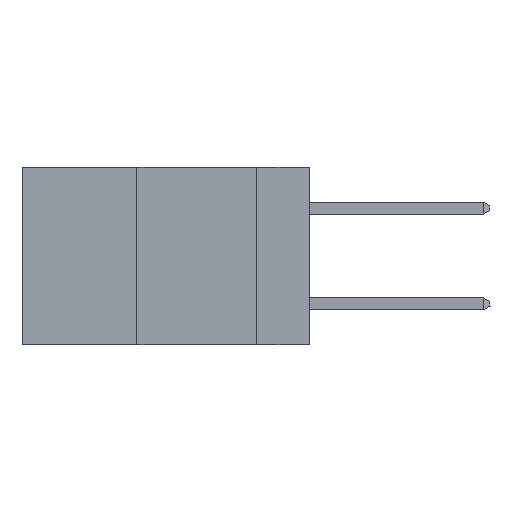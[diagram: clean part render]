
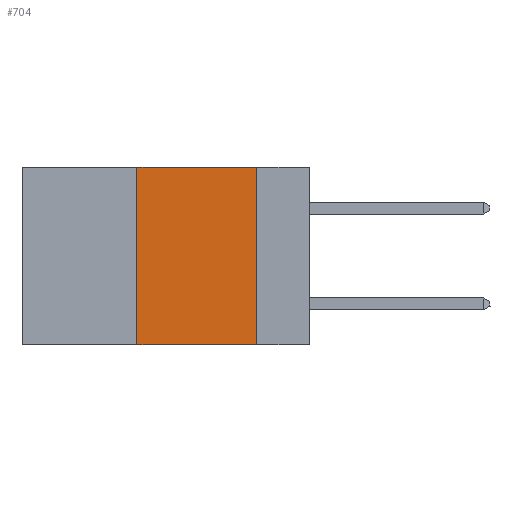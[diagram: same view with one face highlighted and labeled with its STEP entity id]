
A CAD part, left-side view. The second image highlights one B-rep face of the part: STEP entity #704.
In plain terms, the highlighted planar face has unit normal (-1, 0, 0).
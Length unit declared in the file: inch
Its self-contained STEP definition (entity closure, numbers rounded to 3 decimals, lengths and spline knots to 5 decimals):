
#374 = CARTESIAN_POINT ( 'NONE',  ( 0., 0.11, 0. ) ) ;
#409 = AXIS2_PLACEMENT_3D ( 'NONE', #14676, #9984, #1478 ) ;
#520 = ORIENTED_EDGE ( 'NONE', *, *, #13879, .T. ) ;
#557 = ORIENTED_EDGE ( 'NONE', *, *, #12809, .F. ) ;
#704 = ADVANCED_FACE ( 'NONE', ( #5198 ), #9905, .F. ) ;
#795 = DIRECTION ( 'NONE',  ( 0., 0., -1. ) ) ;
#1293 = EDGE_CURVE ( 'NONE', #7593, #11720, #13810, .T. ) ;
#1335 = VECTOR ( 'NONE', #5170, 39.37008 ) ;
#1478 = DIRECTION ( 'NONE',  ( 0., 0., -1. ) ) ;
#2125 = EDGE_CURVE ( 'NONE', #11720, #12497, #3118, .T. ) ;
#2465 = VECTOR ( 'NONE', #10276, 39.37008 ) ;
#2947 = VECTOR ( 'NONE', #795, 39.37008 ) ;
#3118 = LINE ( 'NONE', #13779, #2947 ) ;
#3247 = DIRECTION ( 'NONE',  ( 0., -1., 0. ) ) ;
#3865 = CARTESIAN_POINT ( 'NONE',  ( 0., 0.36, 0. ) ) ;
#4091 = VECTOR ( 'NONE', #3247, 39.37008 ) ;
#5119 = CARTESIAN_POINT ( 'NONE',  ( 0., 0.11, -0.37 ) ) ;
#5170 = DIRECTION ( 'NONE',  ( 0., 0., 1. ) ) ;
#5198 = FACE_OUTER_BOUND ( 'NONE', #7524, .T. ) ;
#5818 = CARTESIAN_POINT ( 'NONE',  ( 0., 0.36, 0. ) ) ;
#6253 = LINE ( 'NONE', #3865, #1335 ) ;
#6775 = ORIENTED_EDGE ( 'NONE', *, *, #1293, .F. ) ;
#7524 = EDGE_LOOP ( 'NONE', ( #8094, #6775, #557, #520 ) ) ;
#7593 = VERTEX_POINT ( 'NONE', #5818 ) ;
#7931 = CARTESIAN_POINT ( 'NONE',  ( 0., 0.6, 0. ) ) ;
#8094 = ORIENTED_EDGE ( 'NONE', *, *, #2125, .F. ) ;
#9229 = VERTEX_POINT ( 'NONE', #15073 ) ;
#9905 = PLANE ( 'NONE',  #409 ) ;
#9984 = DIRECTION ( 'NONE',  ( 1., 0., 0. ) ) ;
#10276 = DIRECTION ( 'NONE',  ( 0., -1., 0. ) ) ;
#10284 = LINE ( 'NONE', #13893, #4091 ) ;
#11720 = VERTEX_POINT ( 'NONE', #374 ) ;
#12497 = VERTEX_POINT ( 'NONE', #5119 ) ;
#12809 = EDGE_CURVE ( 'NONE', #9229, #7593, #6253, .T. ) ;
#13779 = CARTESIAN_POINT ( 'NONE',  ( 0., 0.11, 0. ) ) ;
#13810 = LINE ( 'NONE', #7931, #2465 ) ;
#13879 = EDGE_CURVE ( 'NONE', #9229, #12497, #10284, .T. ) ;
#13893 = CARTESIAN_POINT ( 'NONE',  ( 0., 0.6, -0.37 ) ) ;
#14676 = CARTESIAN_POINT ( 'NONE',  ( 0., 0.6, 0. ) ) ;
#15073 = CARTESIAN_POINT ( 'NONE',  ( 0., 0.36, -0.37 ) ) ;
